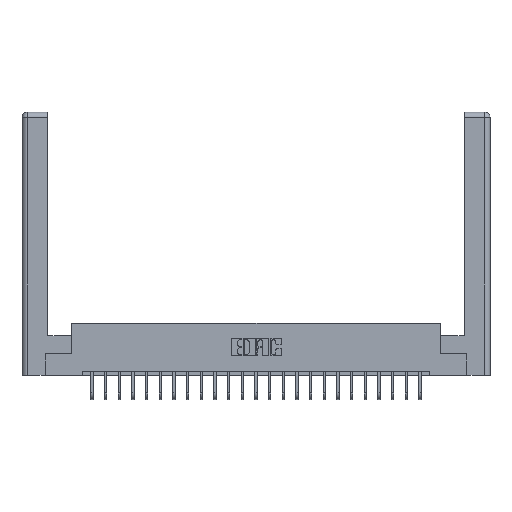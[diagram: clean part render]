
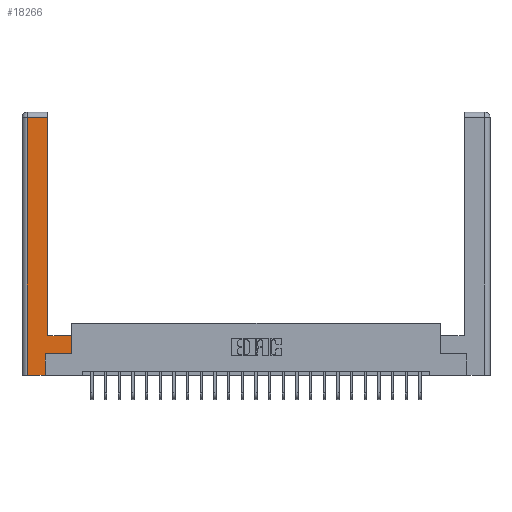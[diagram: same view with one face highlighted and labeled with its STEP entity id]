
A CAD part, top view. The second image highlights one B-rep face of the part: STEP entity #18266.
In plain terms, the highlighted planar face has unit normal (0, 0, 1).
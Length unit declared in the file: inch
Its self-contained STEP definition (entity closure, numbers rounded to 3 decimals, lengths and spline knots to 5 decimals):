
#55 = EDGE_LOOP ( 'NONE', ( #10548, #18042, #21604, #5313, #21871, #21507, #16191, #2098 ) ) ;
#463 = EDGE_CURVE ( 'NONE', #18276, #15902, #7271, .T. ) ;
#639 = CARTESIAN_POINT ( 'NONE',  ( 0., 0., 0. ) ) ;
#958 = LINE ( 'NONE', #20410, #14833 ) ;
#1195 = CARTESIAN_POINT ( 'NONE',  ( 0.565, 0.45, 0. ) ) ;
#1879 = LINE ( 'NONE', #1195, #20039 ) ;
#2098 = ORIENTED_EDGE ( 'NONE', *, *, #9540, .T. ) ;
#2230 = CARTESIAN_POINT ( 'NONE',  ( 0.295, 0.45, 0. ) ) ;
#2309 = DIRECTION ( 'NONE',  ( -1., 0., 0. ) ) ;
#2486 = CARTESIAN_POINT ( 'NONE',  ( 0.0615, 0., 0. ) ) ;
#2613 = DIRECTION ( 'NONE',  ( 1., 0., 0. ) ) ;
#3056 = LINE ( 'NONE', #15186, #22596 ) ;
#3829 = EDGE_CURVE ( 'NONE', #4368, #20671, #9922, .T. ) ;
#4148 = LINE ( 'NONE', #18303, #5306 ) ;
#4368 = VERTEX_POINT ( 'NONE', #8729 ) ;
#4842 = DIRECTION ( 'NONE',  ( 0., 1., 0. ) ) ;
#5306 = VECTOR ( 'NONE', #12932, 39.37008 ) ;
#5313 = ORIENTED_EDGE ( 'NONE', *, *, #19709, .T. ) ;
#5870 = AXIS2_PLACEMENT_3D ( 'NONE', #639, #14817, #2309 ) ;
#6457 = DIRECTION ( 'NONE',  ( 0., 1., 0. ) ) ;
#7089 = CARTESIAN_POINT ( 'NONE',  ( 0.0615, 0., 0. ) ) ;
#7202 = LINE ( 'NONE', #20904, #10925 ) ;
#7271 = LINE ( 'NONE', #10746, #17481 ) ;
#7380 = DIRECTION ( 'NONE',  ( -1., 0., 0. ) ) ;
#7495 = EDGE_CURVE ( 'NONE', #21562, #18276, #7202, .T. ) ;
#7714 = CARTESIAN_POINT ( 'NONE',  ( 0.265, 0.245, 0. ) ) ;
#8729 = CARTESIAN_POINT ( 'NONE',  ( 0.295, 2.94, 0. ) ) ;
#9140 = CARTESIAN_POINT ( 'NONE',  ( 0.0615, 2.94, 0. ) ) ;
#9540 = EDGE_CURVE ( 'NONE', #18600, #13493, #4148, .T. ) ;
#9922 = LINE ( 'NONE', #9140, #16453 ) ;
#10437 = EDGE_CURVE ( 'NONE', #15902, #18600, #1879, .T. ) ;
#10548 = ORIENTED_EDGE ( 'NONE', *, *, #21486, .T. ) ;
#10746 = CARTESIAN_POINT ( 'NONE',  ( 0.565, 0.245, 0. ) ) ;
#10925 = VECTOR ( 'NONE', #15505, 39.37008 ) ;
#11227 = PLANE ( 'NONE',  #5870 ) ;
#12932 = DIRECTION ( 'NONE',  ( -1., 0., 0. ) ) ;
#13493 = VERTEX_POINT ( 'NONE', #2230 ) ;
#13845 = CARTESIAN_POINT ( 'NONE',  ( 0.265, 0., 0. ) ) ;
#14780 = VERTEX_POINT ( 'NONE', #2486 ) ;
#14817 = DIRECTION ( 'NONE',  ( 0., 0., -1. ) ) ;
#14833 = VECTOR ( 'NONE', #6457, 39.37008 ) ;
#14852 = CARTESIAN_POINT ( 'NONE',  ( 0.565, 0.245, 0. ) ) ;
#14941 = CARTESIAN_POINT ( 'NONE',  ( 0.0615, 2.94, 0. ) ) ;
#15186 = CARTESIAN_POINT ( 'NONE',  ( 0.265, 0., 0. ) ) ;
#15505 = DIRECTION ( 'NONE',  ( 0., 1., 0. ) ) ;
#15902 = VERTEX_POINT ( 'NONE', #14852 ) ;
#16109 = DIRECTION ( 'NONE',  ( 1., 0., 0. ) ) ;
#16191 = ORIENTED_EDGE ( 'NONE', *, *, #10437, .T. ) ;
#16193 = LINE ( 'NONE', #7089, #19876 ) ;
#16453 = VECTOR ( 'NONE', #7380, 39.37008 ) ;
#17481 = VECTOR ( 'NONE', #16109, 39.37008 ) ;
#18004 = EDGE_CURVE ( 'NONE', #20671, #14780, #16193, .T. ) ;
#18042 = ORIENTED_EDGE ( 'NONE', *, *, #3829, .T. ) ;
#18266 = ADVANCED_FACE ( 'NONE', ( #21308 ), #11227, .F. ) ;
#18276 = VERTEX_POINT ( 'NONE', #7714 ) ;
#18303 = CARTESIAN_POINT ( 'NONE',  ( 0.295, 0.45, 0. ) ) ;
#18600 = VERTEX_POINT ( 'NONE', #21492 ) ;
#19709 = EDGE_CURVE ( 'NONE', #14780, #21562, #3056, .T. ) ;
#19876 = VECTOR ( 'NONE', #23419, 39.37008 ) ;
#20039 = VECTOR ( 'NONE', #4842, 39.37008 ) ;
#20410 = CARTESIAN_POINT ( 'NONE',  ( 0.295, 3., 0. ) ) ;
#20671 = VERTEX_POINT ( 'NONE', #14941 ) ;
#20904 = CARTESIAN_POINT ( 'NONE',  ( 0.265, 0.245, 0. ) ) ;
#21308 = FACE_OUTER_BOUND ( 'NONE', #55, .T. ) ;
#21486 = EDGE_CURVE ( 'NONE', #13493, #4368, #958, .T. ) ;
#21492 = CARTESIAN_POINT ( 'NONE',  ( 0.565, 0.45, 0. ) ) ;
#21507 = ORIENTED_EDGE ( 'NONE', *, *, #463, .T. ) ;
#21562 = VERTEX_POINT ( 'NONE', #13845 ) ;
#21604 = ORIENTED_EDGE ( 'NONE', *, *, #18004, .T. ) ;
#21871 = ORIENTED_EDGE ( 'NONE', *, *, #7495, .T. ) ;
#22596 = VECTOR ( 'NONE', #2613, 39.37008 ) ;
#23419 = DIRECTION ( 'NONE',  ( 0., -1., 0. ) ) ;
